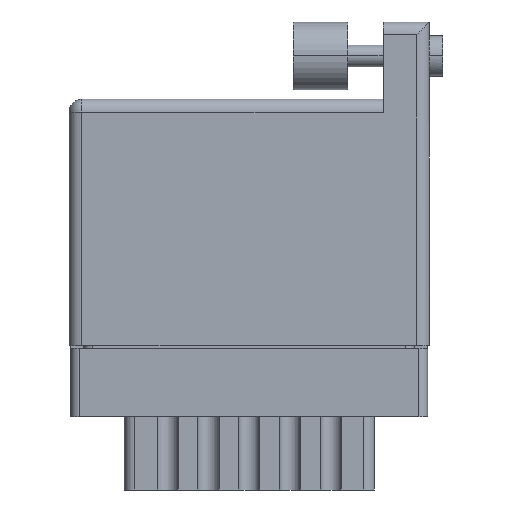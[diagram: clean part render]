
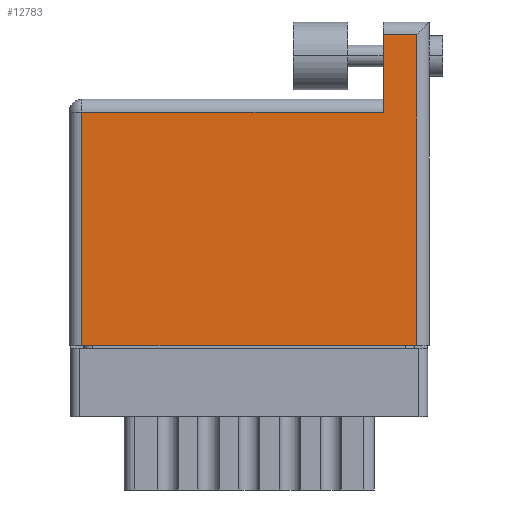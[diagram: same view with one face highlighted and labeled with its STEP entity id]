
A CAD part, front view. The second image highlights one B-rep face of the part: STEP entity #12783.
In plain terms, the highlighted face is planar.
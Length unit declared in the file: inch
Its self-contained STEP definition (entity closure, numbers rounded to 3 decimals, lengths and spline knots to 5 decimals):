
#599 = CARTESIAN_POINT ( 'NONE',  ( 1.278, 0., 0. ) ) ;
#1066 = DIRECTION ( 'NONE',  ( 1., 0., 0. ) ) ;
#2455 = VERTEX_POINT ( 'NONE', #599 ) ;
#2975 = VERTEX_POINT ( 'NONE', #20000 ) ;
#3473 = CARTESIAN_POINT ( 'NONE',  ( 0.047, 0., 0. ) ) ;
#3694 = EDGE_CURVE ( 'NONE', #2455, #13974, #17242, .T. ) ;
#3726 = EDGE_CURVE ( 'NONE', #13974, #9369, #12038, .T. ) ;
#4179 = ORIENTED_EDGE ( 'NONE', *, *, #3726, .T. ) ;
#4419 = ORIENTED_EDGE ( 'NONE', *, *, #7911, .T. ) ;
#4561 = EDGE_CURVE ( 'NONE', #11759, #9787, #21361, .T. ) ;
#4625 = DIRECTION ( 'NONE',  ( -1., 0., 0. ) ) ;
#4751 = CARTESIAN_POINT ( 'NONE',  ( 0., 0.906, 0. ) ) ;
#4980 = EDGE_LOOP ( 'NONE', ( #17957, #10867, #4179, #10411, #19077, #4419 ) ) ;
#4985 = CARTESIAN_POINT ( 'NONE',  ( 1.155, 1.19, 0. ) ) ;
#5305 = DIRECTION ( 'NONE',  ( 0., -1., 0. ) ) ;
#5422 = LINE ( 'NONE', #20187, #21859 ) ;
#5447 = FACE_OUTER_BOUND ( 'NONE', #4980, .T. ) ;
#6052 = EDGE_CURVE ( 'NONE', #2975, #2455, #5422, .T. ) ;
#7096 = CARTESIAN_POINT ( 'NONE',  ( 0.047, 0.859, 0. ) ) ;
#7697 = VECTOR ( 'NONE', #19002, 39.37008 ) ;
#7911 = EDGE_CURVE ( 'NONE', #9787, #2975, #13003, .T. ) ;
#8128 = DIRECTION ( 'NONE',  ( 0., 1., 0. ) ) ;
#9369 = VERTEX_POINT ( 'NONE', #9585 ) ;
#9585 = CARTESIAN_POINT ( 'NONE',  ( 1.155, 1.143, 0. ) ) ;
#9787 = VERTEX_POINT ( 'NONE', #7096 ) ;
#9798 = CARTESIAN_POINT ( 'NONE',  ( 1.278, 1.19, 0. ) ) ;
#10411 = ORIENTED_EDGE ( 'NONE', *, *, #22526, .T. ) ;
#10711 = VECTOR ( 'NONE', #4625, 39.37008 ) ;
#10867 = ORIENTED_EDGE ( 'NONE', *, *, #3694, .T. ) ;
#11759 = VERTEX_POINT ( 'NONE', #15321 ) ;
#12038 = LINE ( 'NONE', #16977, #10711 ) ;
#12783 = ADVANCED_FACE ( 'NONE', ( #5447 ), #18764, .F. ) ;
#13003 = LINE ( 'NONE', #3473, #17659 ) ;
#13504 = CARTESIAN_POINT ( 'NONE',  ( 1.278, 1.143, 0. ) ) ;
#13974 = VERTEX_POINT ( 'NONE', #13504 ) ;
#14199 = VECTOR ( 'NONE', #18679, 39.37008 ) ;
#15192 = AXIS2_PLACEMENT_3D ( 'NONE', #4751, #20558, #16873 ) ;
#15321 = CARTESIAN_POINT ( 'NONE',  ( 1.155, 0.859, 0. ) ) ;
#16873 = DIRECTION ( 'NONE',  ( -1., 0., 0. ) ) ;
#16977 = CARTESIAN_POINT ( 'NONE',  ( 1.155, 1.143, 0. ) ) ;
#17242 = LINE ( 'NONE', #9798, #20586 ) ;
#17659 = VECTOR ( 'NONE', #5305, 39.37008 ) ;
#17957 = ORIENTED_EDGE ( 'NONE', *, *, #6052, .T. ) ;
#18679 = DIRECTION ( 'NONE',  ( -1., 0., 0. ) ) ;
#18764 = PLANE ( 'NONE',  #15192 ) ;
#19002 = DIRECTION ( 'NONE',  ( 0., -1., 0. ) ) ;
#19077 = ORIENTED_EDGE ( 'NONE', *, *, #4561, .T. ) ;
#20000 = CARTESIAN_POINT ( 'NONE',  ( 0.047, 0., 0. ) ) ;
#20187 = CARTESIAN_POINT ( 'NONE',  ( 0., 0., 0. ) ) ;
#20557 = LINE ( 'NONE', #4985, #7697 ) ;
#20558 = DIRECTION ( 'NONE',  ( 0., 0., -1. ) ) ;
#20586 = VECTOR ( 'NONE', #8128, 39.37008 ) ;
#21361 = LINE ( 'NONE', #22478, #14199 ) ;
#21859 = VECTOR ( 'NONE', #1066, 39.37008 ) ;
#22478 = CARTESIAN_POINT ( 'NONE',  ( 0., 0.859, 0. ) ) ;
#22526 = EDGE_CURVE ( 'NONE', #9369, #11759, #20557, .T. ) ;
